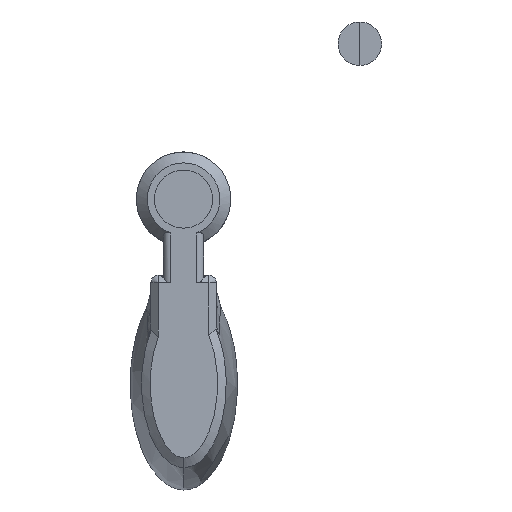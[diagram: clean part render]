
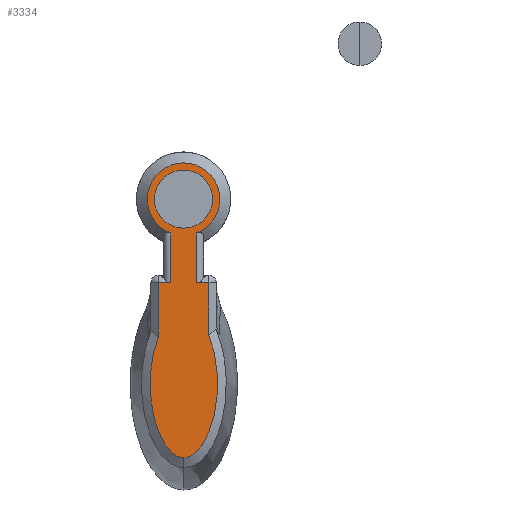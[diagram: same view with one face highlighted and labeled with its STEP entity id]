
A CAD part, left-side view. The second image highlights one B-rep face of the part: STEP entity #3334.
In plain terms, the highlighted planar face has unit normal (-1, 0, 0).
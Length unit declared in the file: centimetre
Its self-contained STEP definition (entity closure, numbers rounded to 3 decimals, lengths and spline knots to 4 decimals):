
#51=FACE_BOUND($,#555,.T.);
#88=CIRCLE($,#3557,0.5);
#89=CIRCLE($,#3558,0.4);
#169=B_SPLINE_CURVE_WITH_KNOTS($,3,(#5919,#5920,#5921,#5922,#5923,#5924,
#5925,#5926,#5927,#5928,#5929,#5930,#5931,#5932),.UNSPECIFIED.,.F.,.F.,
(4,1,1,1,1,1,1,1,1,1,1,4),(-0.1205,0.0089,0.1382,
0.397,0.4293,0.4617,0.5264,
0.591,0.6234,0.6557,1.1732,1.6464),
 .UNSPECIFIED.);
#170=B_SPLINE_CURVE_WITH_KNOTS($,3,(#5934,#5935,#5936,#5937,#5938,#5939,
#5940,#5941,#5942,#5943,#5944,#5945,#5946,#5947,#5948,#5949,#5950),
 .UNSPECIFIED.,.F.,.F.,(4,1,1,1,1,1,1,2,1,1,1,2,4),(3.1012,3.4004,
3.7412,4.0819,4.2523,4.4227,4.5931,
4.7634,4.8106,4.8342,4.8578,4.8813,
4.8815),.UNSPECIFIED.);
#355=FACE_OUTER_BOUND($,#554,.T.);
#554=EDGE_LOOP($,(#2853,#2854,#2855,#2856,#2857,#2858,#2859,#2860,#2861));
#555=EDGE_LOOP($,(#2862));
#914=LINE($,#5886,#1250);
#916=LINE($,#5915,#1252);
#917=LINE($,#5917,#1253);
#918=LINE($,#5952,#1254);
#919=LINE($,#5954,#1255);
#920=LINE($,#5955,#1256);
#1250=VECTOR($,#4278,0.6835);
#1252=VECTOR($,#4284,0.17);
#1253=VECTOR($,#4285,0.7503);
#1254=VECTOR($,#4286,0.7291);
#1255=VECTOR($,#4287,0.17);
#1256=VECTOR($,#4288,0.6835);
#1544=VERTEX_POINT($,#5883);
#1545=VERTEX_POINT($,#5885);
#1548=VERTEX_POINT($,#5912);
#1549=VERTEX_POINT($,#5914);
#1550=VERTEX_POINT($,#5916);
#1551=VERTEX_POINT($,#5918);
#1552=VERTEX_POINT($,#5933);
#1553=VERTEX_POINT($,#5951);
#1554=VERTEX_POINT($,#5953);
#1555=VERTEX_POINT($,#5956);
#1990=EDGE_CURVE($,#1544,#1545,#914,.T.);
#1994=EDGE_CURVE($,#1545,#1548,#88,.T.);
#1995=EDGE_CURVE($,#1549,#1544,#916,.T.);
#1996=EDGE_CURVE($,#1550,#1549,#917,.T.);
#1997=EDGE_CURVE($,#1551,#1550,#169,.T.);
#1998=EDGE_CURVE($,#1552,#1551,#170,.T.);
#1999=EDGE_CURVE($,#1553,#1552,#918,.T.);
#2000=EDGE_CURVE($,#1554,#1553,#919,.T.);
#2001=EDGE_CURVE($,#1548,#1554,#920,.T.);
#2002=EDGE_CURVE($,#1555,#1555,#89,.T.);
#2853=ORIENTED_EDGE($,*,*,#1994,.F.);
#2854=ORIENTED_EDGE($,*,*,#1990,.F.);
#2855=ORIENTED_EDGE($,*,*,#1995,.F.);
#2856=ORIENTED_EDGE($,*,*,#1996,.F.);
#2857=ORIENTED_EDGE($,*,*,#1997,.F.);
#2858=ORIENTED_EDGE($,*,*,#1998,.F.);
#2859=ORIENTED_EDGE($,*,*,#1999,.F.);
#2860=ORIENTED_EDGE($,*,*,#2000,.F.);
#2861=ORIENTED_EDGE($,*,*,#2001,.F.);
#2862=ORIENTED_EDGE($,*,*,#2002,.F.);
#3175=PLANE($,#3556);
#3334=ADVANCED_FACE($,(#355,#51),#3175,.F.);
#3556=AXIS2_PLACEMENT_3D($,#5911,#4280,#4281);
#3557=AXIS2_PLACEMENT_3D($,#5913,#4282,#4283);
#3558=AXIS2_PLACEMENT_3D($,#5957,#4289,#4290);
#4278=DIRECTION($,(0.,0.,1.));
#4280=DIRECTION('center_axis',(1.,0.,0.));
#4281=DIRECTION('ref_axis',(0.,0.,1.));
#4282=DIRECTION('center_axis',(1.,0.,0.));
#4283=DIRECTION('ref_axis',(0.,0.,
-1.));
#4284=DIRECTION($,(0.,-1.,0.));
#4285=DIRECTION($,(0.,0.,1.));
#4286=DIRECTION($,(0.,0.,-1.));
#4287=DIRECTION($,(0.,-1.,0.));
#4288=DIRECTION($,(0.,0.,-1.));
#4289=DIRECTION('center_axis',(-1.,0.,0.));
#4290=DIRECTION('ref_axis',(0.,0.,
-1.));
#5883=CARTESIAN_POINT('',(6.0679,4.9629,-3.2221));
#5885=CARTESIAN_POINT('',(6.0679,4.9629,-2.5385));
#5886=CARTESIAN_POINT($,(6.0679,4.9629,-2.5971));
#5911=CARTESIAN_POINT('Origin',(6.0679,4.7829,-2.1221));
#5912=CARTESIAN_POINT('',(6.0679,4.6029,-2.5385));
#5913=CARTESIAN_POINT('Origin',(6.0679,4.7829,-2.0721));
#5914=CARTESIAN_POINT('',(6.0679,5.1329,-3.2221));
#5915=CARTESIAN_POINT($,(6.0679,4.7829,-3.2221));
#5916=CARTESIAN_POINT('',(6.0679,5.133,-3.9724));
#5917=CARTESIAN_POINT($,(6.0679,5.1329,-2.1221));
#5918=CARTESIAN_POINT('',(6.0679,4.7787,-5.6329));
#5919=CARTESIAN_POINT('Ctrl Pts',(6.0679,4.7787,-5.6329));
#5920=CARTESIAN_POINT('Ctrl Pts',(6.0679,4.8068,-5.6329));
#5921=CARTESIAN_POINT('Ctrl Pts',(6.0679,4.8622,-5.6207));
#5922=CARTESIAN_POINT('Ctrl Pts',(6.0679,4.9738,-5.545));
#5923=CARTESIAN_POINT('Ctrl Pts',(6.0679,5.0466,-5.4421));
#5924=CARTESIAN_POINT('Ctrl Pts',(6.0679,5.0931,-5.3514));
#5925=CARTESIAN_POINT('Ctrl Pts',(6.0679,5.1112,-5.3132));
#5926=CARTESIAN_POINT('Ctrl Pts',(6.0679,5.1325,-5.2628));
#5927=CARTESIAN_POINT('Ctrl Pts',(6.0679,5.152,-5.2087));
#5928=CARTESIAN_POINT('Ctrl Pts',(6.0679,5.1663,-5.1637));
#5929=CARTESIAN_POINT('Ctrl Pts',(6.0679,5.2274,-4.9543));
#5930=CARTESIAN_POINT('Ctrl Pts',(6.0679,5.2717,-4.5163));
#5931=CARTESIAN_POINT('Ctrl Pts',(6.0679,5.1911,-4.1231));
#5932=CARTESIAN_POINT('Ctrl Pts',(6.0679,5.1329,-3.9724));
#5933=CARTESIAN_POINT('',(6.0679,4.4329,-3.9512));
#5934=CARTESIAN_POINT('Ctrl Pts',(6.0679,4.4329,-3.9512));
#5935=CARTESIAN_POINT('Ctrl Pts',(6.0679,4.3948,-4.0446));
#5936=CARTESIAN_POINT('Ctrl Pts',(6.0679,4.3297,-4.2765));
#5937=CARTESIAN_POINT('Ctrl Pts',(6.0679,4.3014,-4.6871));
#5938=CARTESIAN_POINT('Ctrl Pts',(6.0679,4.3495,-5.0387));
#5939=CARTESIAN_POINT('Ctrl Pts',(6.0679,4.428,-5.2794));
#5940=CARTESIAN_POINT('Ctrl Pts',(6.0679,4.4994,-5.4251));
#5941=CARTESIAN_POINT('Ctrl Pts',(6.0679,4.591,-5.5485));
#5942=CARTESIAN_POINT('Ctrl Pts',(6.0679,4.6649,-5.6018));
#5943=CARTESIAN_POINT('Ctrl Pts',(6.0679,4.7125,-5.6213));
#5944=CARTESIAN_POINT('Ctrl Pts',(6.0679,4.7279,-5.6264));
#5945=CARTESIAN_POINT('Ctrl Pts',(6.0679,4.7482,-5.6306));
#5946=CARTESIAN_POINT('Ctrl Pts',(6.0679,4.7634,-5.6324));
#5947=CARTESIAN_POINT('Ctrl Pts',(6.0679,4.7735,-5.6329));
#5948=CARTESIAN_POINT('Ctrl Pts',(6.0679,4.7787,-5.6329));
#5949=CARTESIAN_POINT('Ctrl Pts',(6.0679,4.7787,-5.6329));
#5950=CARTESIAN_POINT('Ctrl Pts',(6.0679,4.7787,-5.6329));
#5951=CARTESIAN_POINT('',(6.0679,4.4329,-3.2221));
#5952=CARTESIAN_POINT($,(6.0679,4.4329,-2.1221));
#5953=CARTESIAN_POINT('',(6.0679,4.6029,-3.2221));
#5954=CARTESIAN_POINT($,(6.0679,4.7829,-3.2221));
#5955=CARTESIAN_POINT($,(6.0679,4.6029,-2.5971));
#5956=CARTESIAN_POINT('',(6.0679,4.7829,-1.6721));
#5957=CARTESIAN_POINT('Origin',(6.0679,4.7829,-2.0721));
